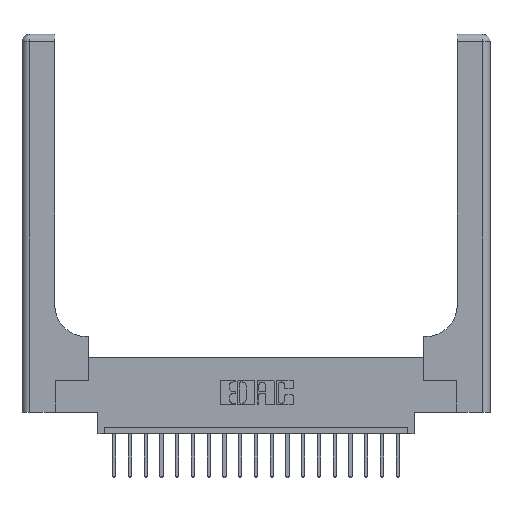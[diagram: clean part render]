
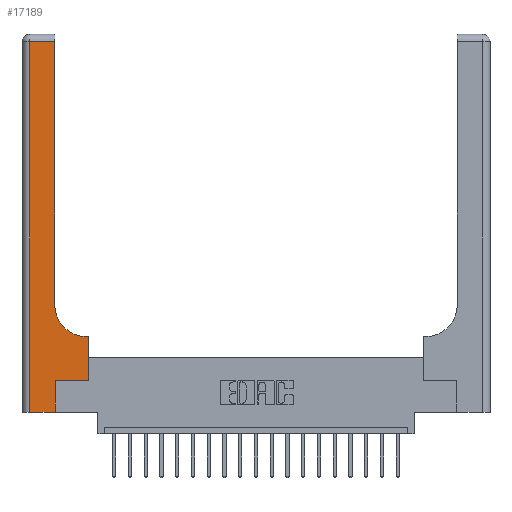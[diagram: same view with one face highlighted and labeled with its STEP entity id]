
A CAD part, top view. The second image highlights one B-rep face of the part: STEP entity #17189.
In plain terms, the highlighted planar face has unit normal (0, 0, 1).
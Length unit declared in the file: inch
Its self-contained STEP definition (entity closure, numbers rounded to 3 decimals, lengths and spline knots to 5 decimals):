
#208 = VECTOR ( 'NONE', #18947, 39.37008 ) ;
#300 = LINE ( 'NONE', #11799, #17673 ) ;
#382 = CARTESIAN_POINT ( 'NONE',  ( 0.528, 0.25, 0.37 ) ) ;
#1395 = CIRCLE ( 'NONE', #20230, 0.25 ) ;
#1523 = DIRECTION ( 'NONE',  ( 0., 0., -1. ) ) ;
#1688 = ORIENTED_EDGE ( 'NONE', *, *, #13739, .T. ) ;
#2029 = CARTESIAN_POINT ( 'NONE',  ( 0.528, 0.6, 0.37 ) ) ;
#2244 = VERTEX_POINT ( 'NONE', #3338 ) ;
#2411 = DIRECTION ( 'NONE',  ( 1., 0., 0. ) ) ;
#2712 = VECTOR ( 'NONE', #17406, 39.37008 ) ;
#2930 = CARTESIAN_POINT ( 'NONE',  ( 0.265, 0.25, 0.37 ) ) ;
#3295 = LINE ( 'NONE', #12166, #15302 ) ;
#3338 = CARTESIAN_POINT ( 'NONE',  ( 0.06, 0., 0.37 ) ) ;
#4208 = ORIENTED_EDGE ( 'NONE', *, *, #6379, .T. ) ;
#4312 = VERTEX_POINT ( 'NONE', #10683 ) ;
#4321 = CARTESIAN_POINT ( 'NONE',  ( 0.26, 3., 0.37 ) ) ;
#4654 = DIRECTION ( 'NONE',  ( -1., 0., 0. ) ) ;
#5380 = VERTEX_POINT ( 'NONE', #10954 ) ;
#6064 = VERTEX_POINT ( 'NONE', #2029 ) ;
#6189 = LINE ( 'NONE', #4321, #17199 ) ;
#6379 = EDGE_CURVE ( 'NONE', #2244, #8862, #300, .T. ) ;
#6427 = EDGE_LOOP ( 'NONE', ( #1688, #12260, #18933, #4208, #8022, #10743, #11677, #6544, #9380 ) ) ;
#6467 = CARTESIAN_POINT ( 'NONE',  ( 0.26, 0.6, 0.37 ) ) ;
#6544 = ORIENTED_EDGE ( 'NONE', *, *, #16131, .T. ) ;
#6898 = CARTESIAN_POINT ( 'NONE',  ( 0.51, 0.85, 0.37 ) ) ;
#7324 = LINE ( 'NONE', #6467, #208 ) ;
#7409 = CARTESIAN_POINT ( 'NONE',  ( 0.51, 0.6, 0.37 ) ) ;
#7450 = CARTESIAN_POINT ( 'NONE',  ( 0., 2.94, 0.37 ) ) ;
#7462 = DIRECTION ( 'NONE',  ( 0., 1., 0. ) ) ;
#7580 = VERTEX_POINT ( 'NONE', #2930 ) ;
#8022 = ORIENTED_EDGE ( 'NONE', *, *, #18207, .T. ) ;
#8571 = EDGE_CURVE ( 'NONE', #7580, #16840, #18095, .T. ) ;
#8862 = VERTEX_POINT ( 'NONE', #12031 ) ;
#9380 = ORIENTED_EDGE ( 'NONE', *, *, #19707, .T. ) ;
#10385 = DIRECTION ( 'NONE',  ( 0., 1., 0. ) ) ;
#10683 = CARTESIAN_POINT ( 'NONE',  ( 0.06, 2.94, 0.37 ) ) ;
#10743 = ORIENTED_EDGE ( 'NONE', *, *, #8571, .T. ) ;
#10831 = PLANE ( 'NONE',  #13584 ) ;
#10899 = CARTESIAN_POINT ( 'NONE',  ( 0., 3., 0.37 ) ) ;
#10954 = CARTESIAN_POINT ( 'NONE',  ( 0.26, 0.85, 0.37 ) ) ;
#11156 = VECTOR ( 'NONE', #10385, 39.37008 ) ;
#11677 = ORIENTED_EDGE ( 'NONE', *, *, #13386, .T. ) ;
#11799 = CARTESIAN_POINT ( 'NONE',  ( 0., 0., 0.37 ) ) ;
#12031 = CARTESIAN_POINT ( 'NONE',  ( 0.265, 0., 0.37 ) ) ;
#12160 = EDGE_CURVE ( 'NONE', #15081, #4312, #15687, .T. ) ;
#12166 = CARTESIAN_POINT ( 'NONE',  ( 0.06, 3., 0.37 ) ) ;
#12260 = ORIENTED_EDGE ( 'NONE', *, *, #12160, .T. ) ;
#12458 = EDGE_CURVE ( 'NONE', #4312, #2244, #3295, .T. ) ;
#12530 = CARTESIAN_POINT ( 'NONE',  ( 0.265, 0.25, 0.37 ) ) ;
#13005 = DIRECTION ( 'NONE',  ( 0., 0., -1. ) ) ;
#13035 = DIRECTION ( 'NONE',  ( 0., 1., 0. ) ) ;
#13386 = EDGE_CURVE ( 'NONE', #16840, #6064, #17915, .T. ) ;
#13584 = AXIS2_PLACEMENT_3D ( 'NONE', #10899, #1523, #4654 ) ;
#13739 = EDGE_CURVE ( 'NONE', #5380, #15081, #6189, .T. ) ;
#15081 = VERTEX_POINT ( 'NONE', #19422 ) ;
#15302 = VECTOR ( 'NONE', #19895, 39.37008 ) ;
#15687 = LINE ( 'NONE', #7450, #20235 ) ;
#15863 = FACE_OUTER_BOUND ( 'NONE', #6427, .T. ) ;
#16131 = EDGE_CURVE ( 'NONE', #6064, #17031, #7324, .T. ) ;
#16251 = CARTESIAN_POINT ( 'NONE',  ( 0.528, 0.25, 0.37 ) ) ;
#16840 = VERTEX_POINT ( 'NONE', #16251 ) ;
#17031 = VERTEX_POINT ( 'NONE', #7409 ) ;
#17189 = ADVANCED_FACE ( 'NONE', ( #15863 ), #10831, .F. ) ;
#17199 = VECTOR ( 'NONE', #7462, 39.37008 ) ;
#17258 = LINE ( 'NONE', #18137, #11156 ) ;
#17406 = DIRECTION ( 'NONE',  ( 1., 0., 0. ) ) ;
#17636 = DIRECTION ( 'NONE',  ( 1., 0., 0. ) ) ;
#17673 = VECTOR ( 'NONE', #2411, 39.37008 ) ;
#17674 = VECTOR ( 'NONE', #13035, 39.37008 ) ;
#17915 = LINE ( 'NONE', #382, #17674 ) ;
#18095 = LINE ( 'NONE', #12530, #2712 ) ;
#18137 = CARTESIAN_POINT ( 'NONE',  ( 0.265, 0., 0.37 ) ) ;
#18207 = EDGE_CURVE ( 'NONE', #8862, #7580, #17258, .T. ) ;
#18353 = DIRECTION ( 'NONE',  ( -1., 0., 0. ) ) ;
#18933 = ORIENTED_EDGE ( 'NONE', *, *, #12458, .T. ) ;
#18947 = DIRECTION ( 'NONE',  ( -1., 0., 0. ) ) ;
#19422 = CARTESIAN_POINT ( 'NONE',  ( 0.26, 2.94, 0.37 ) ) ;
#19707 = EDGE_CURVE ( 'NONE', #17031, #5380, #1395, .T. ) ;
#19895 = DIRECTION ( 'NONE',  ( 0., -1., 0. ) ) ;
#20230 = AXIS2_PLACEMENT_3D ( 'NONE', #6898, #13005, #17636 ) ;
#20235 = VECTOR ( 'NONE', #18353, 39.37008 ) ;
